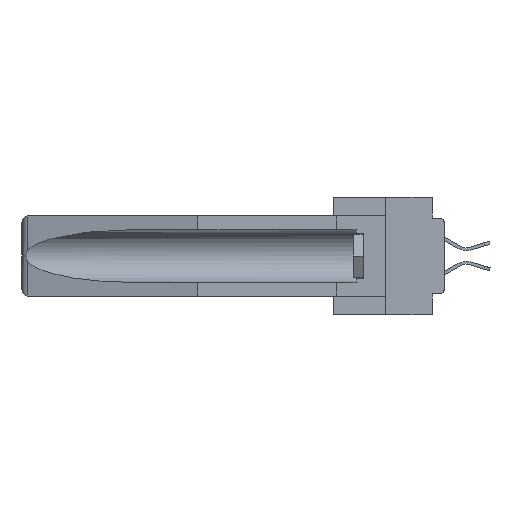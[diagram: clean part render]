
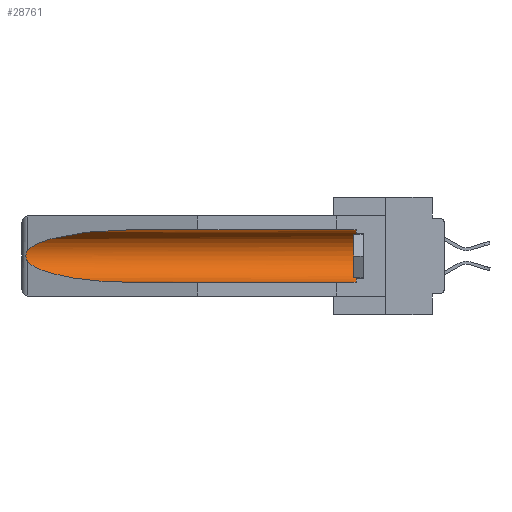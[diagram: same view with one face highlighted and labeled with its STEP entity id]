
A CAD part, left-side view. The second image highlights one B-rep face of the part: STEP entity #28761.
In plain terms, the highlighted cylindrical face has radius 2.857 mm (diameter 5.715 mm), a partial arc.
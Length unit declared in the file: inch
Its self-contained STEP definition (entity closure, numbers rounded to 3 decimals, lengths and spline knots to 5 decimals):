
#857 = CARTESIAN_POINT ( 'NONE',  ( 0.26655, 1.53094, -0.18657 ) ) ;
#1016 = EDGE_CURVE ( 'NONE', #17297, #10509, #28768, .T. ) ;
#1185 = VERTEX_POINT ( 'NONE', #8614 ) ;
#1497 =( BOUNDED_CURVE ( )  B_SPLINE_CURVE ( 3, ( #24948, #3572, #6136, #6030 ),
 .UNSPECIFIED., .F., .F. ) 
 B_SPLINE_CURVE_WITH_KNOTS ( ( 4, 4 ),
 ( 0.1948, 1.5708 ),
 .UNSPECIFIED. ) 
 CURVE ( )  GEOMETRIC_REPRESENTATION_ITEM ( )  RATIONAL_B_SPLINE_CURVE ( ( 1., 0.848, 0.848, 1. ) ) 
 REPRESENTATION_ITEM ( '' )  );
#1807 = CARTESIAN_POINT ( 'NONE',  ( 0.155, -0.30754, -0.1715 ) ) ;
#2400 = DIRECTION ( 'NONE',  ( 0., 1., 0. ) ) ;
#2535 = VERTEX_POINT ( 'NONE', #21103 ) ;
#2702 = CARTESIAN_POINT ( 'NONE',  ( 0.155, -0.30754, -0.059 ) ) ;
#3026 = CARTESIAN_POINT ( 'NONE',  ( 0.26597, 1.5296, -0.19026 ) ) ;
#3245 = CARTESIAN_POINT ( 'NONE',  ( 0.26537, 1.52718, -0.19328 ) ) ;
#3572 = CARTESIAN_POINT ( 'NONE',  ( 0.25451, 1.48313, -0.24835 ) ) ;
#4464 = CARTESIAN_POINT ( 'NONE',  ( 0.155, 1.07973, -0.059 ) ) ;
#4696 = DIRECTION ( 'NONE',  ( 0., 0., 1. ) ) ;
#4699 =( BOUNDED_CURVE ( )  B_SPLINE_CURVE ( 3, ( #26248, #4931, #19266, #7236 ),
 .UNSPECIFIED., .F., .F. ) 
 B_SPLINE_CURVE_WITH_KNOTS ( ( 4, 4 ),
 ( 4.71239, 6.08839 ),
 .UNSPECIFIED. ) 
 CURVE ( )  GEOMETRIC_REPRESENTATION_ITEM ( )  RATIONAL_B_SPLINE_CURVE ( ( 1., 0.848, 0.848, 1. ) ) 
 REPRESENTATION_ITEM ( '' )  );
#4877 = CARTESIAN_POINT ( 'NONE',  ( 0.155, -0.30754, -0.284 ) ) ;
#4931 = CARTESIAN_POINT ( 'NONE',  ( 0.21114, 1.30732, -0.059 ) ) ;
#5049 = VERTEX_POINT ( 'NONE', #18915 ) ;
#5409 = CARTESIAN_POINT ( 'NONE',  ( 0.26597, 1.52961, -0.15275 ) ) ;
#6030 = CARTESIAN_POINT ( 'NONE',  ( 0.155, 1.07973, -0.284 ) ) ;
#6136 = CARTESIAN_POINT ( 'NONE',  ( 0.21114, 1.30732, -0.284 ) ) ;
#6606 = B_SPLINE_CURVE_WITH_KNOTS ( 'NONE', 3,
 ( #17273, #5409, #29071, #29265, #10195, #17475, #12782, #857, #3026, #3245 ),
 .UNSPECIFIED., .F., .F.,
 ( 4, 2, 2, 2, 4 ),
 ( 0., 0.00029, 0.00058, 0.00087, 0.00117 ),
 .UNSPECIFIED. ) ;
#6621 = VECTOR ( 'NONE', #2400, 39.37008 ) ;
#7236 = CARTESIAN_POINT ( 'NONE',  ( 0.26537, 1.52718, -0.14972 ) ) ;
#7428 = ORIENTED_EDGE ( 'NONE', *, *, #1016, .F. ) ;
#8614 = CARTESIAN_POINT ( 'NONE',  ( 0.26537, 1.52718, -0.19328 ) ) ;
#10195 = CARTESIAN_POINT ( 'NONE',  ( 0.2675, 1.53308, -0.16763 ) ) ;
#10509 = VERTEX_POINT ( 'NONE', #25405 ) ;
#10855 = DIRECTION ( 'NONE',  ( 0., -1., 0. ) ) ;
#10917 = EDGE_LOOP ( 'NONE', ( #28769, #18099, #29517, #7428, #19798, #24469 ) ) ;
#10967 = DIRECTION ( 'NONE',  ( 0., 0., 1. ) ) ;
#12782 = CARTESIAN_POINT ( 'NONE',  ( 0.2673, 1.53269, -0.17917 ) ) ;
#14310 = FACE_OUTER_BOUND ( 'NONE', #10917, .T. ) ;
#14666 = DIRECTION ( 'NONE',  ( 0., 1., 0. ) ) ;
#17273 = CARTESIAN_POINT ( 'NONE',  ( 0.26537, 1.52718, -0.14972 ) ) ;
#17297 = VERTEX_POINT ( 'NONE', #21663 ) ;
#17475 = CARTESIAN_POINT ( 'NONE',  ( 0.2675, 1.53308, -0.17534 ) ) ;
#17639 = CYLINDRICAL_SURFACE ( 'NONE', #27884, 0.1125 ) ;
#18099 = ORIENTED_EDGE ( 'NONE', *, *, #22648, .T. ) ;
#18731 = VECTOR ( 'NONE', #14666, 39.37008 ) ;
#18906 = EDGE_CURVE ( 'NONE', #1185, #10509, #1497, .T. ) ;
#18915 = CARTESIAN_POINT ( 'NONE',  ( 0.26537, 1.52718, -0.14972 ) ) ;
#19266 = CARTESIAN_POINT ( 'NONE',  ( 0.25451, 1.48313, -0.09465 ) ) ;
#19271 = VERTEX_POINT ( 'NONE', #4464 ) ;
#19798 = ORIENTED_EDGE ( 'NONE', *, *, #28101, .T. ) ;
#20319 = CARTESIAN_POINT ( 'NONE',  ( 0.155, 0.126, -0.1715 ) ) ;
#20496 = DIRECTION ( 'NONE',  ( 0., 1., 0. ) ) ;
#21103 = CARTESIAN_POINT ( 'NONE',  ( 0.155, 0.126, -0.059 ) ) ;
#21663 = CARTESIAN_POINT ( 'NONE',  ( 0.155, 0.126, -0.284 ) ) ;
#21763 = EDGE_CURVE ( 'NONE', #19271, #5049, #4699, .T. ) ;
#21789 = CIRCLE ( 'NONE', #25496, 0.1125 ) ;
#22648 = EDGE_CURVE ( 'NONE', #5049, #1185, #6606, .T. ) ;
#24469 = ORIENTED_EDGE ( 'NONE', *, *, #30715, .T. ) ;
#24948 = CARTESIAN_POINT ( 'NONE',  ( 0.26537, 1.52718, -0.19328 ) ) ;
#25405 = CARTESIAN_POINT ( 'NONE',  ( 0.155, 1.07973, -0.284 ) ) ;
#25496 = AXIS2_PLACEMENT_3D ( 'NONE', #20319, #10855, #10967 ) ;
#25581 = LINE ( 'NONE', #2702, #6621 ) ;
#26248 = CARTESIAN_POINT ( 'NONE',  ( 0.155, 1.07973, -0.059 ) ) ;
#27884 = AXIS2_PLACEMENT_3D ( 'NONE', #1807, #20496, #4696 ) ;
#28101 = EDGE_CURVE ( 'NONE', #17297, #2535, #21789, .T. ) ;
#28761 = ADVANCED_FACE ( 'NONE', ( #14310 ), #17639, .F. ) ;
#28768 = LINE ( 'NONE', #4877, #18731 ) ;
#28769 = ORIENTED_EDGE ( 'NONE', *, *, #21763, .T. ) ;
#29071 = CARTESIAN_POINT ( 'NONE',  ( 0.26654, 1.53092, -0.15636 ) ) ;
#29265 = CARTESIAN_POINT ( 'NONE',  ( 0.2673, 1.5327, -0.16383 ) ) ;
#29517 = ORIENTED_EDGE ( 'NONE', *, *, #18906, .T. ) ;
#30715 = EDGE_CURVE ( 'NONE', #2535, #19271, #25581, .T. ) ;
